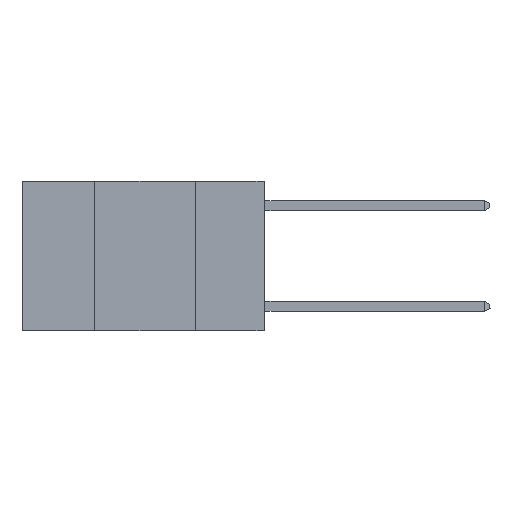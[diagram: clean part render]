
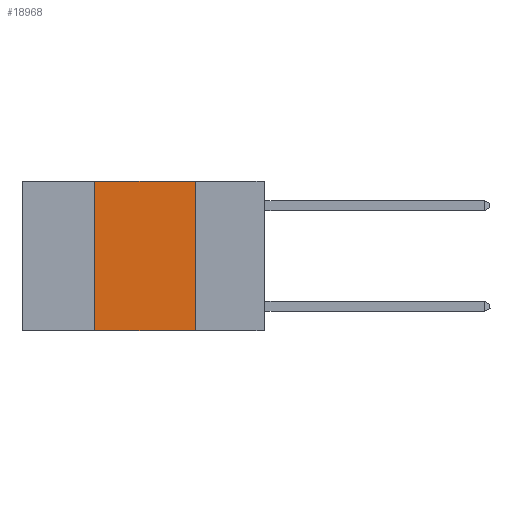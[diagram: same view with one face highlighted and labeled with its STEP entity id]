
A CAD part, left-side view. The second image highlights one B-rep face of the part: STEP entity #18968.
In plain terms, the highlighted planar face has unit normal (-1, 0, 0).
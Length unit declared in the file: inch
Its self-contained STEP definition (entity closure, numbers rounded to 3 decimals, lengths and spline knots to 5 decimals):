
#435 = VECTOR ( 'NONE', #16539, 39.37008 ) ;
#584 = LINE ( 'NONE', #3795, #2090 ) ;
#634 = EDGE_CURVE ( 'NONE', #11223, #7786, #584, .T. ) ;
#1441 = EDGE_CURVE ( 'NONE', #16799, #11223, #13361, .T. ) ;
#2090 = VECTOR ( 'NONE', #6714, 39.37008 ) ;
#2631 = DIRECTION ( 'NONE',  ( 1., 0., 0. ) ) ;
#3795 = CARTESIAN_POINT ( 'NONE',  ( 0., 0.17, 0. ) ) ;
#3873 = CARTESIAN_POINT ( 'NONE',  ( 0., 0.42, -0.37 ) ) ;
#4595 = EDGE_CURVE ( 'NONE', #10479, #16799, #5828, .T. ) ;
#4816 = VECTOR ( 'NONE', #19058, 39.37008 ) ;
#4901 = CARTESIAN_POINT ( 'NONE',  ( 0., 0.17, 0. ) ) ;
#5828 = LINE ( 'NONE', #10646, #17465 ) ;
#6211 = DIRECTION ( 'NONE',  ( 0., 0., -1. ) ) ;
#6714 = DIRECTION ( 'NONE',  ( 0., 0., -1. ) ) ;
#6801 = CARTESIAN_POINT ( 'NONE',  ( 0., 0.6, -0.37 ) ) ;
#7786 = VERTEX_POINT ( 'NONE', #17306 ) ;
#8764 = ORIENTED_EDGE ( 'NONE', *, *, #11693, .T. ) ;
#10265 = FACE_OUTER_BOUND ( 'NONE', #18454, .T. ) ;
#10479 = VERTEX_POINT ( 'NONE', #3873 ) ;
#10646 = CARTESIAN_POINT ( 'NONE',  ( 0., 0.42, 0. ) ) ;
#10663 = CARTESIAN_POINT ( 'NONE',  ( 0., 0.6, 0. ) ) ;
#11223 = VERTEX_POINT ( 'NONE', #4901 ) ;
#11693 = EDGE_CURVE ( 'NONE', #10479, #7786, #14494, .T. ) ;
#13361 = LINE ( 'NONE', #10663, #435 ) ;
#13457 = CARTESIAN_POINT ( 'NONE',  ( 0., 0.42, 0. ) ) ;
#14494 = LINE ( 'NONE', #6801, #4816 ) ;
#14680 = ORIENTED_EDGE ( 'NONE', *, *, #4595, .F. ) ;
#14720 = ORIENTED_EDGE ( 'NONE', *, *, #1441, .F. ) ;
#15203 = AXIS2_PLACEMENT_3D ( 'NONE', #16787, #2631, #6211 ) ;
#16333 = PLANE ( 'NONE',  #15203 ) ;
#16539 = DIRECTION ( 'NONE',  ( 0., -1., 0. ) ) ;
#16787 = CARTESIAN_POINT ( 'NONE',  ( 0., 0.6, 0. ) ) ;
#16799 = VERTEX_POINT ( 'NONE', #13457 ) ;
#17306 = CARTESIAN_POINT ( 'NONE',  ( 0., 0.17, -0.37 ) ) ;
#17465 = VECTOR ( 'NONE', #18207, 39.37008 ) ;
#18207 = DIRECTION ( 'NONE',  ( 0., 0., 1. ) ) ;
#18454 = EDGE_LOOP ( 'NONE', ( #19216, #14720, #14680, #8764 ) ) ;
#18968 = ADVANCED_FACE ( 'NONE', ( #10265 ), #16333, .F. ) ;
#19058 = DIRECTION ( 'NONE',  ( 0., -1., 0. ) ) ;
#19216 = ORIENTED_EDGE ( 'NONE', *, *, #634, .F. ) ;
